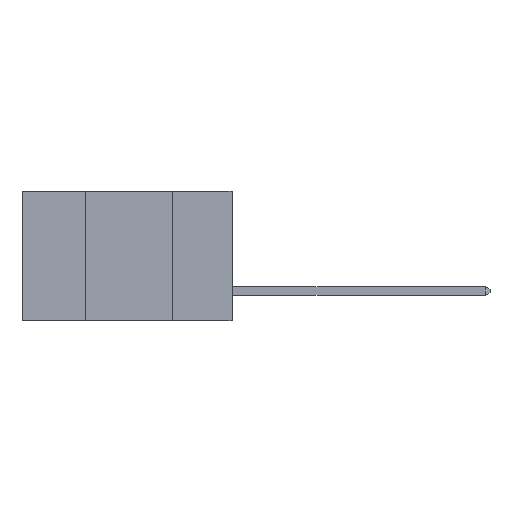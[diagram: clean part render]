
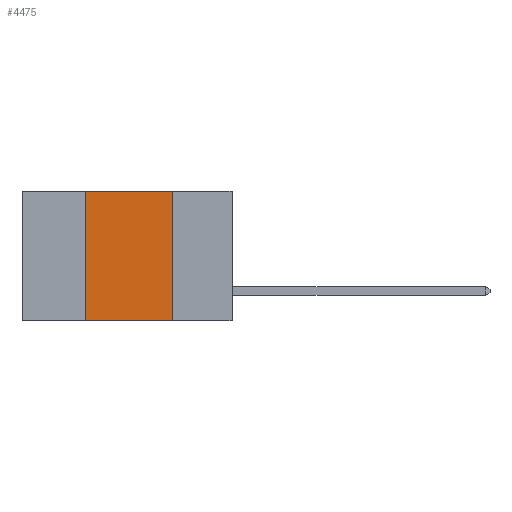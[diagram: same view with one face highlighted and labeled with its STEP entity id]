
A CAD part, left-side view. The second image highlights one B-rep face of the part: STEP entity #4475.
In plain terms, the highlighted planar face has unit normal (-1, 0, 0).
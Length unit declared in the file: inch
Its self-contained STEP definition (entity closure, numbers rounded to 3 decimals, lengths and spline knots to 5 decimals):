
#968 = EDGE_CURVE ( 'NONE', #11351, #31890, #8922, .T. ) ;
#3224 = CARTESIAN_POINT ( 'NONE',  ( 0., 0.6, 0. ) ) ;
#3362 = CARTESIAN_POINT ( 'NONE',  ( 0., 0.6, -0.37 ) ) ;
#4214 = LINE ( 'NONE', #3362, #17015 ) ;
#4387 = EDGE_CURVE ( 'NONE', #31878, #26758, #6252, .T. ) ;
#4475 = ADVANCED_FACE ( 'NONE', ( #9863 ), #26037, .F. ) ;
#5454 = VECTOR ( 'NONE', #23223, 39.37008 ) ;
#5788 = DIRECTION ( 'NONE',  ( 1., 0., 0. ) ) ;
#5946 = DIRECTION ( 'NONE',  ( 0., -1., 0. ) ) ;
#6252 = LINE ( 'NONE', #10417, #5454 ) ;
#8922 = LINE ( 'NONE', #28685, #28435 ) ;
#9863 = FACE_OUTER_BOUND ( 'NONE', #12985, .T. ) ;
#10413 = CARTESIAN_POINT ( 'NONE',  ( 0., 0.42, 0. ) ) ;
#10417 = CARTESIAN_POINT ( 'NONE',  ( 0., 0.17, 0. ) ) ;
#11153 = EDGE_CURVE ( 'NONE', #31890, #31878, #17494, .T. ) ;
#11351 = VERTEX_POINT ( 'NONE', #22029 ) ;
#12846 = CARTESIAN_POINT ( 'NONE',  ( 0., 0.17, 0. ) ) ;
#12985 = EDGE_LOOP ( 'NONE', ( #32450, #18888, #30072, #19056 ) ) ;
#16757 = CARTESIAN_POINT ( 'NONE',  ( 0., 0.17, -0.37 ) ) ;
#17015 = VECTOR ( 'NONE', #5946, 39.37008 ) ;
#17494 = LINE ( 'NONE', #26427, #32613 ) ;
#18888 = ORIENTED_EDGE ( 'NONE', *, *, #11153, .F. ) ;
#19056 = ORIENTED_EDGE ( 'NONE', *, *, #27215, .T. ) ;
#21279 = DIRECTION ( 'NONE',  ( 0., -1., 0. ) ) ;
#22029 = CARTESIAN_POINT ( 'NONE',  ( 0., 0.42, -0.37 ) ) ;
#22514 = AXIS2_PLACEMENT_3D ( 'NONE', #3224, #5788, #23566 ) ;
#23223 = DIRECTION ( 'NONE',  ( 0., 0., -1. ) ) ;
#23566 = DIRECTION ( 'NONE',  ( 0., 0., -1. ) ) ;
#26037 = PLANE ( 'NONE',  #22514 ) ;
#26105 = DIRECTION ( 'NONE',  ( 0., 0., 1. ) ) ;
#26427 = CARTESIAN_POINT ( 'NONE',  ( 0., 0.6, 0. ) ) ;
#26758 = VERTEX_POINT ( 'NONE', #16757 ) ;
#27215 = EDGE_CURVE ( 'NONE', #11351, #26758, #4214, .T. ) ;
#28435 = VECTOR ( 'NONE', #26105, 39.37008 ) ;
#28685 = CARTESIAN_POINT ( 'NONE',  ( 0., 0.42, 0. ) ) ;
#30072 = ORIENTED_EDGE ( 'NONE', *, *, #968, .F. ) ;
#31878 = VERTEX_POINT ( 'NONE', #12846 ) ;
#31890 = VERTEX_POINT ( 'NONE', #10413 ) ;
#32450 = ORIENTED_EDGE ( 'NONE', *, *, #4387, .F. ) ;
#32613 = VECTOR ( 'NONE', #21279, 39.37008 ) ;
